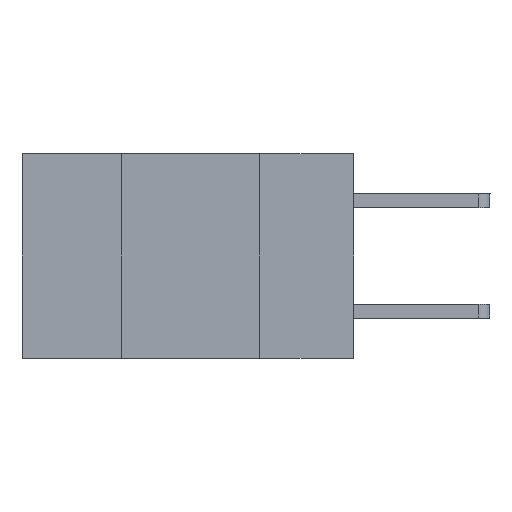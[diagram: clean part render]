
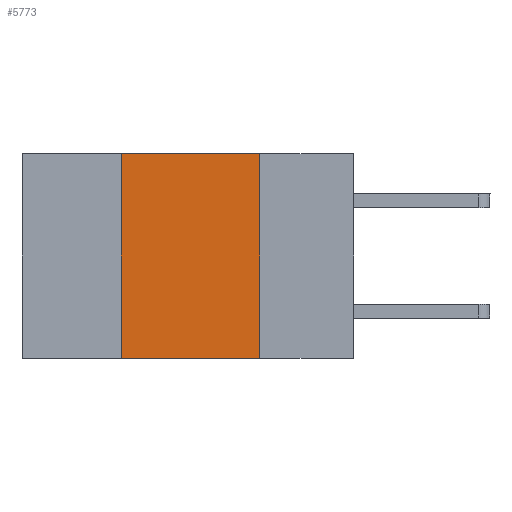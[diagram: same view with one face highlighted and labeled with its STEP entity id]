
A CAD part, left-side view. The second image highlights one B-rep face of the part: STEP entity #5773.
In plain terms, the highlighted planar face has unit normal (-1, 0, 0).
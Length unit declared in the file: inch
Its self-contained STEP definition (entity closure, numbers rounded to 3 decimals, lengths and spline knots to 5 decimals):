
#44 = EDGE_LOOP ( 'NONE', ( #6706, #4110, #4247, #3066 ) ) ;
#210 = CARTESIAN_POINT ( 'NONE',  ( 0., 0.17, -0.37 ) ) ;
#259 = CARTESIAN_POINT ( 'NONE',  ( 0., 0.6, 0. ) ) ;
#344 = CARTESIAN_POINT ( 'NONE',  ( 0., 0.17, 0. ) ) ;
#1038 = VERTEX_POINT ( 'NONE', #7471 ) ;
#1469 = LINE ( 'NONE', #1644, #6285 ) ;
#1644 = CARTESIAN_POINT ( 'NONE',  ( 0., 0.42, 0. ) ) ;
#2130 = EDGE_CURVE ( 'NONE', #1038, #3341, #7425, .T. ) ;
#2148 = EDGE_CURVE ( 'NONE', #3341, #9541, #10607, .T. ) ;
#2227 = VERTEX_POINT ( 'NONE', #10180 ) ;
#2865 = CARTESIAN_POINT ( 'NONE',  ( 0., 0.6, 0. ) ) ;
#3066 = ORIENTED_EDGE ( 'NONE', *, *, #9070, .T. ) ;
#3341 = VERTEX_POINT ( 'NONE', #344 ) ;
#3467 = FACE_OUTER_BOUND ( 'NONE', #44, .T. ) ;
#3490 = CARTESIAN_POINT ( 'NONE',  ( 0., 0.17, 0. ) ) ;
#3855 = PLANE ( 'NONE',  #9816 ) ;
#4110 = ORIENTED_EDGE ( 'NONE', *, *, #2130, .F. ) ;
#4247 = ORIENTED_EDGE ( 'NONE', *, *, #7735, .F. ) ;
#4505 = DIRECTION ( 'NONE',  ( 0., 0., 1. ) ) ;
#4810 = DIRECTION ( 'NONE',  ( 0., 0., -1. ) ) ;
#5773 = ADVANCED_FACE ( 'NONE', ( #3467 ), #3855, .F. ) ;
#6285 = VECTOR ( 'NONE', #4505, 39.37008 ) ;
#6457 = DIRECTION ( 'NONE',  ( 0., -1., 0. ) ) ;
#6706 = ORIENTED_EDGE ( 'NONE', *, *, #2148, .F. ) ;
#7425 = LINE ( 'NONE', #259, #10101 ) ;
#7471 = CARTESIAN_POINT ( 'NONE',  ( 0., 0.42, 0. ) ) ;
#7735 = EDGE_CURVE ( 'NONE', #2227, #1038, #1469, .T. ) ;
#8291 = CARTESIAN_POINT ( 'NONE',  ( 0., 0.6, -0.37 ) ) ;
#9070 = EDGE_CURVE ( 'NONE', #2227, #9541, #9974, .T. ) ;
#9244 = VECTOR ( 'NONE', #10001, 39.37008 ) ;
#9541 = VERTEX_POINT ( 'NONE', #210 ) ;
#9816 = AXIS2_PLACEMENT_3D ( 'NONE', #2865, #10379, #4810 ) ;
#9974 = LINE ( 'NONE', #8291, #12030 ) ;
#10001 = DIRECTION ( 'NONE',  ( 0., 0., -1. ) ) ;
#10101 = VECTOR ( 'NONE', #11729, 39.37008 ) ;
#10180 = CARTESIAN_POINT ( 'NONE',  ( 0., 0.42, -0.37 ) ) ;
#10379 = DIRECTION ( 'NONE',  ( 1., 0., 0. ) ) ;
#10607 = LINE ( 'NONE', #3490, #9244 ) ;
#11729 = DIRECTION ( 'NONE',  ( 0., -1., 0. ) ) ;
#12030 = VECTOR ( 'NONE', #6457, 39.37008 ) ;
